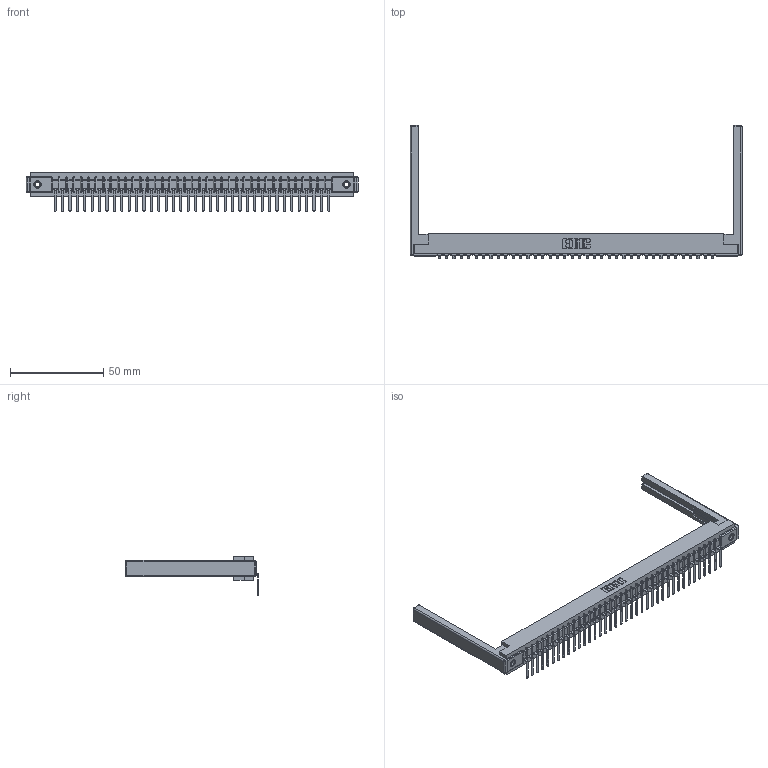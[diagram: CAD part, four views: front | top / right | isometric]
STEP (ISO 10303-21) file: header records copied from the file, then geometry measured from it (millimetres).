
FILE_DESCRIPTION (( 'STEP AP203' ), '1' );
FILE_NAME ('307-038-557-168.STEP', '2019-09-05T09:28:10', ( '' ), ( '' ), 'SwSTEP 2.0', 'SolidWorks 2016', '' );
FILE_SCHEMA (( 'CONFIG_CONTROL_DESIGN' ));
Length unit declared in the file: inch
Products named in the file (5): 307 Part_.156 Dia Mounting Holes; 307-290-002_557; 307-038-557-168; 307-220-068; 345-250-001_345-250-001-102
Assembly tree (43 placements, depth 2):
  307-038-557-168
    307 Part_.156 Dia Mounting Holes
    307-290-002_557  x38
    307-220-068  x2
    345-250-001_345-250-001-102  x2
Bounding box: 178 x 71.29 x 20.66 mm (x, y, z)
Volume: 23498.9 mm3; surface area: 28582.4 mm2
Topology: 43 solids, 43 shells, 3275 faces, 9985 edges, 6530 vertices
Faces by surface type: plane 1944, cylinder 1229, sphere 86, cone 12, torus 4
Entity records: 36683 total; most frequent: CARTESIAN_POINT 6153, ORIENTED_EDGE 6132, DIRECTION 5998, EDGE_CURVE 3066, VECTOR 2344, LINE 2344, VERTEX_POINT 1982, AXIS2_PLACEMENT_3D 1827
